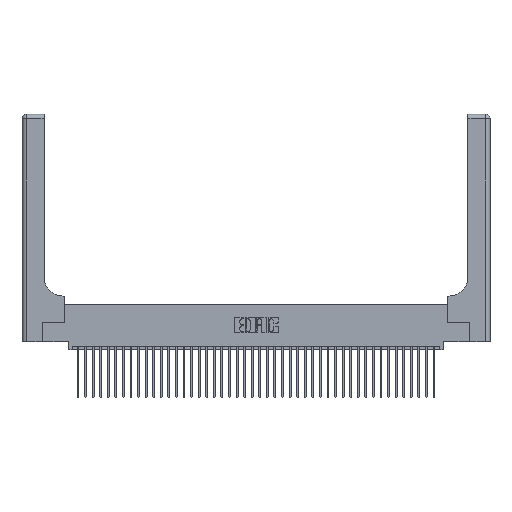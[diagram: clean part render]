
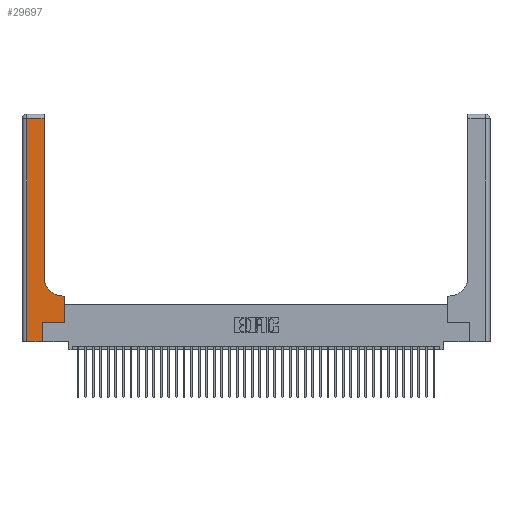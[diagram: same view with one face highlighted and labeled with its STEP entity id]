
A CAD part, top view. The second image highlights one B-rep face of the part: STEP entity #29697.
In plain terms, the highlighted planar face has unit normal (0, 0, 1).
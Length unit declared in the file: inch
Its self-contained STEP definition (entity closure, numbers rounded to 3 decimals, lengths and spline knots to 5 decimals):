
#33 = ORIENTED_EDGE ( 'NONE', *, *, #39884, .T. ) ;
#79 = ORIENTED_EDGE ( 'NONE', *, *, #28276, .T. ) ;
#241 = DIRECTION ( 'NONE',  ( 1., 0., 0. ) ) ;
#651 = CARTESIAN_POINT ( 'NONE',  ( 0.5585, 0.6, 0.37 ) ) ;
#793 = ORIENTED_EDGE ( 'NONE', *, *, #6640, .T. ) ;
#1264 = VECTOR ( 'NONE', #26580, 39.37008 ) ;
#2398 = EDGE_CURVE ( 'NONE', #8096, #31858, #32545, .T. ) ;
#2727 = DIRECTION ( 'NONE',  ( 0., 1., 0. ) ) ;
#2789 = VERTEX_POINT ( 'NONE', #8116 ) ;
#3010 = LINE ( 'NONE', #40848, #18368 ) ;
#3998 = ORIENTED_EDGE ( 'NONE', *, *, #37095, .T. ) ;
#4448 = DIRECTION ( 'NONE',  ( 0., 1., 0. ) ) ;
#4668 = FACE_OUTER_BOUND ( 'NONE', #38551, .T. ) ;
#6379 = VERTEX_POINT ( 'NONE', #9139 ) ;
#6509 = LINE ( 'NONE', #16537, #14218 ) ;
#6640 = EDGE_CURVE ( 'NONE', #23454, #21432, #3010, .T. ) ;
#8096 = VERTEX_POINT ( 'NONE', #25725 ) ;
#8116 = CARTESIAN_POINT ( 'NONE',  ( 0.06, 2.94, 0.37 ) ) ;
#8360 = DIRECTION ( 'NONE',  ( 1., 0., 0. ) ) ;
#9139 = CARTESIAN_POINT ( 'NONE',  ( 0.2915, 2.94, 0.37 ) ) ;
#10019 = DIRECTION ( 'NONE',  ( 0., 0., -1. ) ) ;
#10482 = DIRECTION ( 'NONE',  ( -1., 0., 0. ) ) ;
#10826 = VERTEX_POINT ( 'NONE', #25516 ) ;
#12117 = VECTOR ( 'NONE', #38425, 39.37008 ) ;
#12514 = CARTESIAN_POINT ( 'NONE',  ( 0.2915, 0.6, 0.37 ) ) ;
#13637 = CARTESIAN_POINT ( 'NONE',  ( 0., 3., 0.37 ) ) ;
#13957 = VERTEX_POINT ( 'NONE', #19935 ) ;
#14218 = VECTOR ( 'NONE', #241, 39.37008 ) ;
#14891 = VERTEX_POINT ( 'NONE', #27431 ) ;
#15165 = VECTOR ( 'NONE', #2727, 39.37008 ) ;
#16537 = CARTESIAN_POINT ( 'NONE',  ( 0.269, 0.25, 0.37 ) ) ;
#17995 = LINE ( 'NONE', #33754, #34325 ) ;
#18368 = VECTOR ( 'NONE', #8360, 39.37008 ) ;
#18551 = VECTOR ( 'NONE', #25677, 39.37008 ) ;
#19935 = CARTESIAN_POINT ( 'NONE',  ( 0.5415, 0.6, 0.37 ) ) ;
#20886 = VECTOR ( 'NONE', #33659, 39.37008 ) ;
#21432 = VERTEX_POINT ( 'NONE', #25380 ) ;
#23321 = CARTESIAN_POINT ( 'NONE',  ( 0.06, 3., 0.37 ) ) ;
#23454 = VERTEX_POINT ( 'NONE', #32154 ) ;
#23527 = PLANE ( 'NONE',  #25734 ) ;
#23668 = ORIENTED_EDGE ( 'NONE', *, *, #2398, .T. ) ;
#25380 = CARTESIAN_POINT ( 'NONE',  ( 0.269, 0., 0.37 ) ) ;
#25382 = CARTESIAN_POINT ( 'NONE',  ( 0.2915, 3., 0.37 ) ) ;
#25516 = CARTESIAN_POINT ( 'NONE',  ( 0.269, 0.25, 0.37 ) ) ;
#25677 = DIRECTION ( 'NONE',  ( -1., 0., 0. ) ) ;
#25725 = CARTESIAN_POINT ( 'NONE',  ( 0.5585, 0.25, 0.37 ) ) ;
#25734 = AXIS2_PLACEMENT_3D ( 'NONE', #13637, #30067, #10482 ) ;
#25763 = CARTESIAN_POINT ( 'NONE',  ( 0.5585, 0.25, 0.37 ) ) ;
#26360 = LINE ( 'NONE', #23321, #1264 ) ;
#26580 = DIRECTION ( 'NONE',  ( 0., -1., 0. ) ) ;
#27233 = CARTESIAN_POINT ( 'NONE',  ( 0., 2.94, 0.37 ) ) ;
#27241 = LINE ( 'NONE', #12514, #18551 ) ;
#27431 = CARTESIAN_POINT ( 'NONE',  ( 0.2915, 0.85, 0.37 ) ) ;
#28276 = EDGE_CURVE ( 'NONE', #13957, #14891, #41536, .T. ) ;
#29554 = LINE ( 'NONE', #27233, #20886 ) ;
#29600 = CARTESIAN_POINT ( 'NONE',  ( 0.5415, 0.85, 0.37 ) ) ;
#29697 = ADVANCED_FACE ( 'NONE', ( #4668 ), #23527, .F. ) ;
#29775 = EDGE_CURVE ( 'NONE', #21432, #10826, #17995, .T. ) ;
#30067 = DIRECTION ( 'NONE',  ( 0., 0., -1. ) ) ;
#30613 = ORIENTED_EDGE ( 'NONE', *, *, #37591, .T. ) ;
#31858 = VERTEX_POINT ( 'NONE', #651 ) ;
#31955 = EDGE_CURVE ( 'NONE', #6379, #2789, #29554, .T. ) ;
#32154 = CARTESIAN_POINT ( 'NONE',  ( 0.06, 0., 0.37 ) ) ;
#32545 = LINE ( 'NONE', #25763, #15165 ) ;
#32870 = DIRECTION ( 'NONE',  ( 1., 0., 0. ) ) ;
#33659 = DIRECTION ( 'NONE',  ( -1., 0., 0. ) ) ;
#33754 = CARTESIAN_POINT ( 'NONE',  ( 0.269, 0., 0.37 ) ) ;
#34131 = EDGE_CURVE ( 'NONE', #31858, #13957, #27241, .T. ) ;
#34325 = VECTOR ( 'NONE', #4448, 39.37008 ) ;
#35937 = ORIENTED_EDGE ( 'NONE', *, *, #34131, .T. ) ;
#36306 = AXIS2_PLACEMENT_3D ( 'NONE', #29600, #10019, #32870 ) ;
#36686 = ORIENTED_EDGE ( 'NONE', *, *, #29775, .T. ) ;
#37095 = EDGE_CURVE ( 'NONE', #10826, #8096, #6509, .T. ) ;
#37591 = EDGE_CURVE ( 'NONE', #14891, #6379, #39122, .T. ) ;
#38425 = DIRECTION ( 'NONE',  ( 0., 1., 0. ) ) ;
#38551 = EDGE_LOOP ( 'NONE', ( #30613, #40339, #33, #793, #36686, #3998, #23668, #35937, #79 ) ) ;
#39122 = LINE ( 'NONE', #25382, #12117 ) ;
#39884 = EDGE_CURVE ( 'NONE', #2789, #23454, #26360, .T. ) ;
#40339 = ORIENTED_EDGE ( 'NONE', *, *, #31955, .T. ) ;
#40848 = CARTESIAN_POINT ( 'NONE',  ( 0., 0., 0.37 ) ) ;
#41536 = CIRCLE ( 'NONE', #36306, 0.25 ) ;
